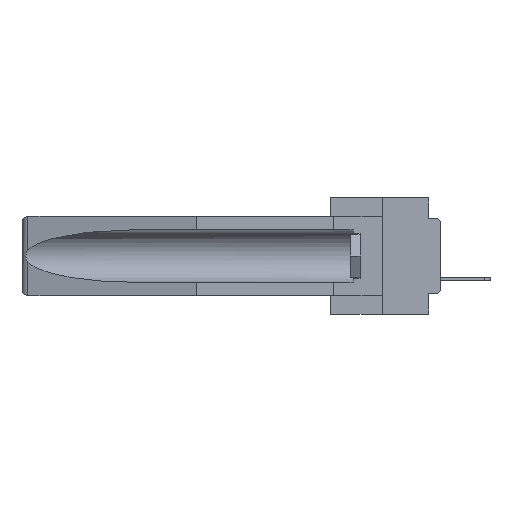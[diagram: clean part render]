
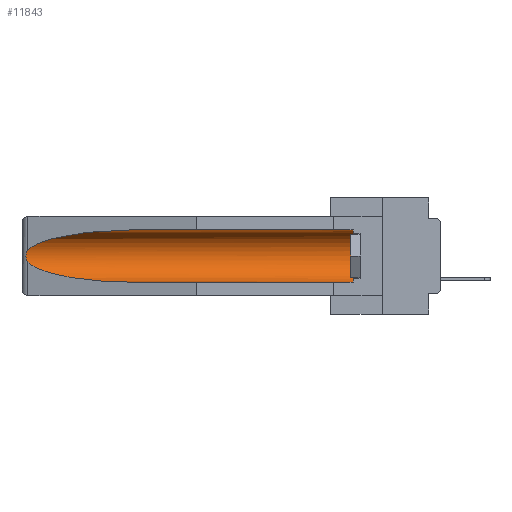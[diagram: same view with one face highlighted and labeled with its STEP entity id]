
A CAD part, left-side view. The second image highlights one B-rep face of the part: STEP entity #11843.
In plain terms, the highlighted cylindrical face has radius 2.857 mm (diameter 5.715 mm), a partial arc.
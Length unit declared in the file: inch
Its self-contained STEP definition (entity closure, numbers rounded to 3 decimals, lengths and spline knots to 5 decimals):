
#467 = DIRECTION ( 'NONE',  ( 0., 1., 0. ) ) ;
#1347 = LINE ( 'NONE', #5329, #8698 ) ;
#1523 = VERTEX_POINT ( 'NONE', #11619 ) ;
#2038 = DIRECTION ( 'NONE',  ( 0., 1., 0. ) ) ;
#2149 = CARTESIAN_POINT ( 'NONE',  ( 0.155, -0.30754, -0.1715 ) ) ;
#2208 = CARTESIAN_POINT ( 'NONE',  ( 0.25451, 1.48313, -0.24835 ) ) ;
#2276 = VERTEX_POINT ( 'NONE', #13148 ) ;
#3366 = VERTEX_POINT ( 'NONE', #12507 ) ;
#3427 = ORIENTED_EDGE ( 'NONE', *, *, #7763, .T. ) ;
#4157 = ORIENTED_EDGE ( 'NONE', *, *, #16548, .T. ) ;
#4612 = EDGE_LOOP ( 'NONE', ( #6821, #19763, #3427, #5017, #29041, #4157 ) ) ;
#5017 = ORIENTED_EDGE ( 'NONE', *, *, #24152, .F. ) ;
#5329 = CARTESIAN_POINT ( 'NONE',  ( 0.155, -0.30754, -0.059 ) ) ;
#5464 = CIRCLE ( 'NONE', #16328, 0.1125 ) ;
#5965 = EDGE_CURVE ( 'NONE', #1523, #2276, #27003, .T. ) ;
#6821 = ORIENTED_EDGE ( 'NONE', *, *, #5965, .T. ) ;
#7655 = CARTESIAN_POINT ( 'NONE',  ( 0.155, -0.30754, -0.284 ) ) ;
#7763 = EDGE_CURVE ( 'NONE', #3366, #20998, #24454, .T. ) ;
#8143 = CARTESIAN_POINT ( 'NONE',  ( 0.2673, 1.5327, -0.16383 ) ) ;
#8253 = CARTESIAN_POINT ( 'NONE',  ( 0.26537, 1.52718, -0.14972 ) ) ;
#8358 = CARTESIAN_POINT ( 'NONE',  ( 0.26655, 1.53094, -0.18657 ) ) ;
#8698 = VECTOR ( 'NONE', #467, 39.37008 ) ;
#9663 = CARTESIAN_POINT ( 'NONE',  ( 0.25451, 1.48313, -0.09465 ) ) ;
#10325 = CARTESIAN_POINT ( 'NONE',  ( 0.155, 1.07973, -0.284 ) ) ;
#11150 = CARTESIAN_POINT ( 'NONE',  ( 0.155, 0.126, -0.284 ) ) ;
#11619 = CARTESIAN_POINT ( 'NONE',  ( 0.155, 1.07973, -0.059 ) ) ;
#11709 = CARTESIAN_POINT ( 'NONE',  ( 0.21114, 1.30732, -0.284 ) ) ;
#11843 = ADVANCED_FACE ( 'NONE', ( #13969 ), #25482, .F. ) ;
#12483 = LINE ( 'NONE', #7655, #17846 ) ;
#12507 = CARTESIAN_POINT ( 'NONE',  ( 0.26537, 1.52718, -0.19328 ) ) ;
#13148 = CARTESIAN_POINT ( 'NONE',  ( 0.26537, 1.52718, -0.14972 ) ) ;
#13406 = CARTESIAN_POINT ( 'NONE',  ( 0.26654, 1.53092, -0.15636 ) ) ;
#13969 = FACE_OUTER_BOUND ( 'NONE', #4612, .T. ) ;
#15057 = CARTESIAN_POINT ( 'NONE',  ( 0.155, 0.126, -0.059 ) ) ;
#15866 = CARTESIAN_POINT ( 'NONE',  ( 0.26597, 1.5296, -0.19026 ) ) ;
#16328 = AXIS2_PLACEMENT_3D ( 'NONE', #21960, #27233, #31807 ) ;
#16548 = EDGE_CURVE ( 'NONE', #31463, #1523, #1347, .T. ) ;
#17846 = VECTOR ( 'NONE', #27427, 39.37008 ) ;
#18229 = CARTESIAN_POINT ( 'NONE',  ( 0.2675, 1.53308, -0.17534 ) ) ;
#18758 = B_SPLINE_CURVE_WITH_KNOTS ( 'NONE', 3,
 ( #8253, #22818, #13406, #8143, #27672, #18229, #27900, #8358, #15866, #25302 ),
 .UNSPECIFIED., .F., .F.,
 ( 4, 2, 2, 2, 4 ),
 ( 0., 0.00029, 0.00058, 0.00087, 0.00117 ),
 .UNSPECIFIED. ) ;
#19763 = ORIENTED_EDGE ( 'NONE', *, *, #29161, .T. ) ;
#20998 = VERTEX_POINT ( 'NONE', #10325 ) ;
#21677 = CARTESIAN_POINT ( 'NONE',  ( 0.155, 1.07973, -0.284 ) ) ;
#21960 = CARTESIAN_POINT ( 'NONE',  ( 0.155, 0.126, -0.1715 ) ) ;
#21983 = CARTESIAN_POINT ( 'NONE',  ( 0.155, 1.07973, -0.059 ) ) ;
#22055 = VERTEX_POINT ( 'NONE', #11150 ) ;
#22818 = CARTESIAN_POINT ( 'NONE',  ( 0.26597, 1.52961, -0.15275 ) ) ;
#24152 = EDGE_CURVE ( 'NONE', #22055, #20998, #12483, .T. ) ;
#24454 =( BOUNDED_CURVE ( )  B_SPLINE_CURVE ( 3, ( #26837, #2208, #11709, #21677 ),
 .UNSPECIFIED., .F., .F. ) 
 B_SPLINE_CURVE_WITH_KNOTS ( ( 4, 4 ),
 ( 0.1948, 1.5708 ),
 .UNSPECIFIED. ) 
 CURVE ( )  GEOMETRIC_REPRESENTATION_ITEM ( )  RATIONAL_B_SPLINE_CURVE ( ( 1., 0.848, 0.848, 1. ) ) 
 REPRESENTATION_ITEM ( '' )  );
#25302 = CARTESIAN_POINT ( 'NONE',  ( 0.26537, 1.52718, -0.19328 ) ) ;
#25482 = CYLINDRICAL_SURFACE ( 'NONE', #29716, 0.1125 ) ;
#26307 = CARTESIAN_POINT ( 'NONE',  ( 0.21114, 1.30732, -0.059 ) ) ;
#26837 = CARTESIAN_POINT ( 'NONE',  ( 0.26537, 1.52718, -0.19328 ) ) ;
#26841 = CARTESIAN_POINT ( 'NONE',  ( 0.26537, 1.52718, -0.14972 ) ) ;
#27003 =( BOUNDED_CURVE ( )  B_SPLINE_CURVE ( 3, ( #21983, #26307, #9663, #26841 ),
 .UNSPECIFIED., .F., .F. ) 
 B_SPLINE_CURVE_WITH_KNOTS ( ( 4, 4 ),
 ( 4.71239, 6.08839 ),
 .UNSPECIFIED. ) 
 CURVE ( )  GEOMETRIC_REPRESENTATION_ITEM ( )  RATIONAL_B_SPLINE_CURVE ( ( 1., 0.848, 0.848, 1. ) ) 
 REPRESENTATION_ITEM ( '' )  );
#27233 = DIRECTION ( 'NONE',  ( 0., -1., 0. ) ) ;
#27427 = DIRECTION ( 'NONE',  ( 0., 1., 0. ) ) ;
#27672 = CARTESIAN_POINT ( 'NONE',  ( 0.2675, 1.53308, -0.16763 ) ) ;
#27900 = CARTESIAN_POINT ( 'NONE',  ( 0.2673, 1.53269, -0.17917 ) ) ;
#29041 = ORIENTED_EDGE ( 'NONE', *, *, #29504, .T. ) ;
#29161 = EDGE_CURVE ( 'NONE', #2276, #3366, #18758, .T. ) ;
#29405 = DIRECTION ( 'NONE',  ( 0., 0., 1. ) ) ;
#29504 = EDGE_CURVE ( 'NONE', #22055, #31463, #5464, .T. ) ;
#29716 = AXIS2_PLACEMENT_3D ( 'NONE', #2149, #2038, #29405 ) ;
#31463 = VERTEX_POINT ( 'NONE', #15057 ) ;
#31807 = DIRECTION ( 'NONE',  ( 0., 0., 1. ) ) ;
